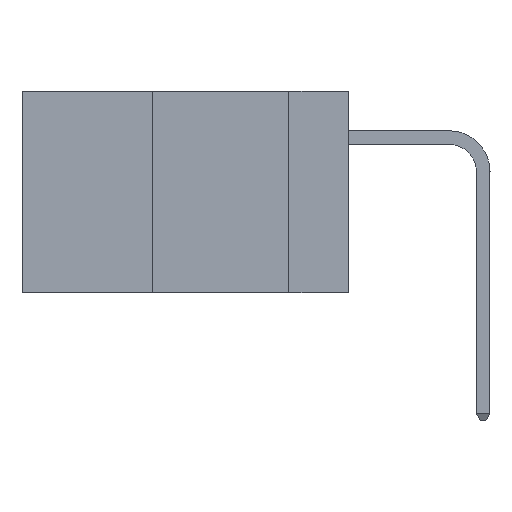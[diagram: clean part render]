
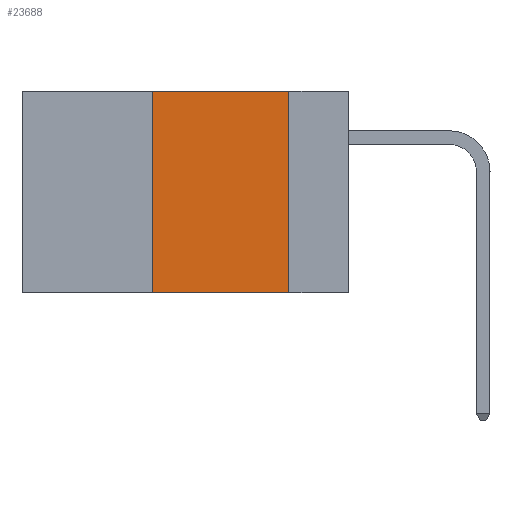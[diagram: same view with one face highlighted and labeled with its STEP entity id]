
A CAD part, left-side view. The second image highlights one B-rep face of the part: STEP entity #23688.
In plain terms, the highlighted planar face has unit normal (-1, 0, 0).
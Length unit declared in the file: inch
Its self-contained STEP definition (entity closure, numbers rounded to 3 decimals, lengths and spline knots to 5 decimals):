
#1 = ORIENTED_EDGE ( 'NONE', *, *, #13411, .F. ) ;
#1332 = CARTESIAN_POINT ( 'NONE',  ( 0., 0.6, 0. ) ) ;
#1574 = VERTEX_POINT ( 'NONE', #13356 ) ;
#1587 = PLANE ( 'NONE',  #17459 ) ;
#2658 = EDGE_CURVE ( 'NONE', #14607, #1574, #11070, .T. ) ;
#3149 = CARTESIAN_POINT ( 'NONE',  ( 0., 0.36, 0. ) ) ;
#4474 = ORIENTED_EDGE ( 'NONE', *, *, #15739, .F. ) ;
#5135 = DIRECTION ( 'NONE',  ( 0., 0., -1. ) ) ;
#6279 = DIRECTION ( 'NONE',  ( 0., 0., -1. ) ) ;
#6851 = FACE_OUTER_BOUND ( 'NONE', #9534, .T. ) ;
#7497 = VERTEX_POINT ( 'NONE', #8516 ) ;
#8516 = CARTESIAN_POINT ( 'NONE',  ( 0., 0.36, 0. ) ) ;
#9055 = DIRECTION ( 'NONE',  ( 1., 0., 0. ) ) ;
#9534 = EDGE_LOOP ( 'NONE', ( #4474, #1, #14590, #12619 ) ) ;
#9955 = LINE ( 'NONE', #17415, #12387 ) ;
#10497 = CARTESIAN_POINT ( 'NONE',  ( 0., 0.36, -0.37 ) ) ;
#10751 = DIRECTION ( 'NONE',  ( 0., 0., 1. ) ) ;
#11070 = LINE ( 'NONE', #21964, #14773 ) ;
#11192 = DIRECTION ( 'NONE',  ( 0., -1., 0. ) ) ;
#12237 = VERTEX_POINT ( 'NONE', #23050 ) ;
#12387 = VECTOR ( 'NONE', #6279, 39.37008 ) ;
#12619 = ORIENTED_EDGE ( 'NONE', *, *, #2658, .T. ) ;
#13356 = CARTESIAN_POINT ( 'NONE',  ( 0., 0.11, -0.37 ) ) ;
#13411 = EDGE_CURVE ( 'NONE', #7497, #12237, #22445, .T. ) ;
#14590 = ORIENTED_EDGE ( 'NONE', *, *, #24057, .F. ) ;
#14607 = VERTEX_POINT ( 'NONE', #10497 ) ;
#14773 = VECTOR ( 'NONE', #18405, 39.37008 ) ;
#14861 = CARTESIAN_POINT ( 'NONE',  ( 0., 0.6, 0. ) ) ;
#15739 = EDGE_CURVE ( 'NONE', #12237, #1574, #9955, .T. ) ;
#17378 = VECTOR ( 'NONE', #11192, 39.37008 ) ;
#17415 = CARTESIAN_POINT ( 'NONE',  ( 0., 0.11, 0. ) ) ;
#17459 = AXIS2_PLACEMENT_3D ( 'NONE', #1332, #9055, #5135 ) ;
#18405 = DIRECTION ( 'NONE',  ( 0., -1., 0. ) ) ;
#21757 = LINE ( 'NONE', #3149, #21785 ) ;
#21785 = VECTOR ( 'NONE', #10751, 39.37008 ) ;
#21964 = CARTESIAN_POINT ( 'NONE',  ( 0., 0.6, -0.37 ) ) ;
#22445 = LINE ( 'NONE', #14861, #17378 ) ;
#23050 = CARTESIAN_POINT ( 'NONE',  ( 0., 0.11, 0. ) ) ;
#23688 = ADVANCED_FACE ( 'NONE', ( #6851 ), #1587, .F. ) ;
#24057 = EDGE_CURVE ( 'NONE', #14607, #7497, #21757, .T. ) ;
